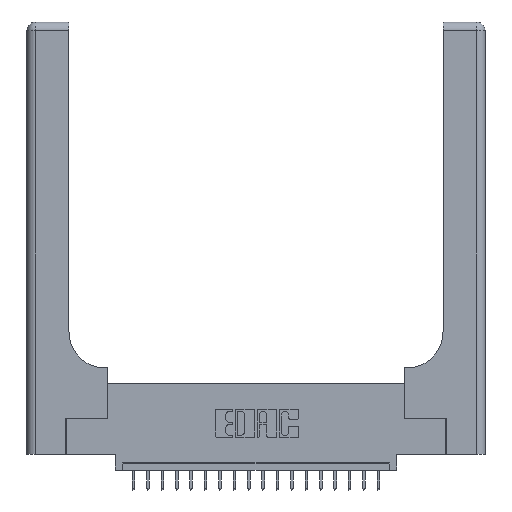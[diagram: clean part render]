
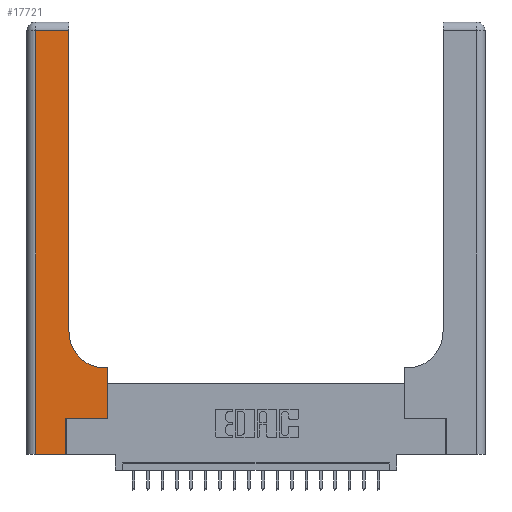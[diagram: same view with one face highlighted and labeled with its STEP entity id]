
A CAD part, top view. The second image highlights one B-rep face of the part: STEP entity #17721.
In plain terms, the highlighted planar face has unit normal (0, 0, 1).
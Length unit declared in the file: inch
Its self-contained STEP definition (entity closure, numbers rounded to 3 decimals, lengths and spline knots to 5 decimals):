
#44 = DIRECTION ( 'NONE',  ( 1., 0., 0. ) ) ;
#94 = ORIENTED_EDGE ( 'NONE', *, *, #19838, .T. ) ;
#142 = ORIENTED_EDGE ( 'NONE', *, *, #20214, .T. ) ;
#247 = LINE ( 'NONE', #5430, #18707 ) ;
#322 = CARTESIAN_POINT ( 'NONE',  ( 0.06, 2.94, 0.37 ) ) ;
#357 = CARTESIAN_POINT ( 'NONE',  ( 0., 3., 0.37 ) ) ;
#572 = CARTESIAN_POINT ( 'NONE',  ( 0.06, 0., 0.37 ) ) ;
#816 = LINE ( 'NONE', #19548, #12916 ) ;
#1489 = DIRECTION ( 'NONE',  ( -1., 0., 0. ) ) ;
#1506 = LINE ( 'NONE', #11626, #2488 ) ;
#1648 = CARTESIAN_POINT ( 'NONE',  ( 0., 2.94, 0.37 ) ) ;
#2311 = EDGE_CURVE ( 'NONE', #4590, #13778, #13427, .T. ) ;
#2370 = EDGE_CURVE ( 'NONE', #12164, #9624, #9039, .T. ) ;
#2488 = VECTOR ( 'NONE', #16895, 39.37008 ) ;
#2582 = VECTOR ( 'NONE', #8360, 39.37008 ) ;
#3870 = CARTESIAN_POINT ( 'NONE',  ( 0.269, 0.25, 0.37 ) ) ;
#4042 = CARTESIAN_POINT ( 'NONE',  ( 0.2915, 2.94, 0.37 ) ) ;
#4059 = CARTESIAN_POINT ( 'NONE',  ( 0.5585, 0.6, 0.37 ) ) ;
#4149 = EDGE_CURVE ( 'NONE', #12044, #16024, #247, .T. ) ;
#4590 = VERTEX_POINT ( 'NONE', #18530 ) ;
#4635 = VERTEX_POINT ( 'NONE', #4042 ) ;
#4765 = CARTESIAN_POINT ( 'NONE',  ( 0.06, 3., 0.37 ) ) ;
#4850 = EDGE_CURVE ( 'NONE', #9624, #4635, #7943, .T. ) ;
#4871 = DIRECTION ( 'NONE',  ( 0., -1., 0. ) ) ;
#4919 = LINE ( 'NONE', #1648, #21273 ) ;
#5108 = AXIS2_PLACEMENT_3D ( 'NONE', #15780, #17350, #44 ) ;
#5430 = CARTESIAN_POINT ( 'NONE',  ( 0.269, 0., 0.37 ) ) ;
#5775 = DIRECTION ( 'NONE',  ( 1., 0., 0. ) ) ;
#6158 = DIRECTION ( 'NONE',  ( 0., 1., 0. ) ) ;
#6850 = EDGE_CURVE ( 'NONE', #13778, #12164, #13624, .T. ) ;
#7212 = DIRECTION ( 'NONE',  ( -1., 0., 0. ) ) ;
#7317 = VECTOR ( 'NONE', #1489, 39.37008 ) ;
#7642 = DIRECTION ( 'NONE',  ( 0., 0., -1. ) ) ;
#7943 = LINE ( 'NONE', #21507, #21957 ) ;
#8293 = EDGE_CURVE ( 'NONE', #4635, #14091, #4919, .T. ) ;
#8360 = DIRECTION ( 'NONE',  ( 0., 1., 0. ) ) ;
#8497 = AXIS2_PLACEMENT_3D ( 'NONE', #357, #7642, #7212 ) ;
#8994 = PLANE ( 'NONE',  #8497 ) ;
#9039 = CIRCLE ( 'NONE', #5108, 0.25 ) ;
#9624 = VERTEX_POINT ( 'NONE', #14130 ) ;
#9705 = ORIENTED_EDGE ( 'NONE', *, *, #8293, .T. ) ;
#10037 = CARTESIAN_POINT ( 'NONE',  ( 0.2915, 0.6, 0.37 ) ) ;
#11086 = VECTOR ( 'NONE', #4871, 39.37008 ) ;
#11626 = CARTESIAN_POINT ( 'NONE',  ( 0., 0., 0.37 ) ) ;
#11823 = LINE ( 'NONE', #4765, #11086 ) ;
#12044 = VERTEX_POINT ( 'NONE', #20009 ) ;
#12164 = VERTEX_POINT ( 'NONE', #16082 ) ;
#12916 = VECTOR ( 'NONE', #5775, 39.37008 ) ;
#13349 = DIRECTION ( 'NONE',  ( -1., 0., 0. ) ) ;
#13427 = LINE ( 'NONE', #15012, #2582 ) ;
#13624 = LINE ( 'NONE', #10037, #7317 ) ;
#13778 = VERTEX_POINT ( 'NONE', #4059 ) ;
#14091 = VERTEX_POINT ( 'NONE', #322 ) ;
#14130 = CARTESIAN_POINT ( 'NONE',  ( 0.2915, 0.85, 0.37 ) ) ;
#14839 = EDGE_CURVE ( 'NONE', #14091, #14942, #11823, .T. ) ;
#14942 = VERTEX_POINT ( 'NONE', #572 ) ;
#15012 = CARTESIAN_POINT ( 'NONE',  ( 0.5585, 0.25, 0.37 ) ) ;
#15015 = ORIENTED_EDGE ( 'NONE', *, *, #4850, .T. ) ;
#15780 = CARTESIAN_POINT ( 'NONE',  ( 0.5415, 0.85, 0.37 ) ) ;
#16024 = VERTEX_POINT ( 'NONE', #3870 ) ;
#16082 = CARTESIAN_POINT ( 'NONE',  ( 0.5415, 0.6, 0.37 ) ) ;
#16293 = ORIENTED_EDGE ( 'NONE', *, *, #2370, .T. ) ;
#16895 = DIRECTION ( 'NONE',  ( 1., 0., 0. ) ) ;
#17161 = EDGE_LOOP ( 'NONE', ( #15015, #9705, #17863, #94, #21268, #142, #19730, #17844, #16293 ) ) ;
#17350 = DIRECTION ( 'NONE',  ( 0., 0., -1. ) ) ;
#17654 = FACE_OUTER_BOUND ( 'NONE', #17161, .T. ) ;
#17721 = ADVANCED_FACE ( 'NONE', ( #17654 ), #8994, .F. ) ;
#17844 = ORIENTED_EDGE ( 'NONE', *, *, #6850, .T. ) ;
#17863 = ORIENTED_EDGE ( 'NONE', *, *, #14839, .T. ) ;
#18530 = CARTESIAN_POINT ( 'NONE',  ( 0.5585, 0.25, 0.37 ) ) ;
#18707 = VECTOR ( 'NONE', #19109, 39.37008 ) ;
#19109 = DIRECTION ( 'NONE',  ( 0., 1., 0. ) ) ;
#19548 = CARTESIAN_POINT ( 'NONE',  ( 0.269, 0.25, 0.37 ) ) ;
#19730 = ORIENTED_EDGE ( 'NONE', *, *, #2311, .T. ) ;
#19838 = EDGE_CURVE ( 'NONE', #14942, #12044, #1506, .T. ) ;
#20009 = CARTESIAN_POINT ( 'NONE',  ( 0.269, 0., 0.37 ) ) ;
#20214 = EDGE_CURVE ( 'NONE', #16024, #4590, #816, .T. ) ;
#21268 = ORIENTED_EDGE ( 'NONE', *, *, #4149, .T. ) ;
#21273 = VECTOR ( 'NONE', #13349, 39.37008 ) ;
#21507 = CARTESIAN_POINT ( 'NONE',  ( 0.2915, 3., 0.37 ) ) ;
#21957 = VECTOR ( 'NONE', #6158, 39.37008 ) ;
